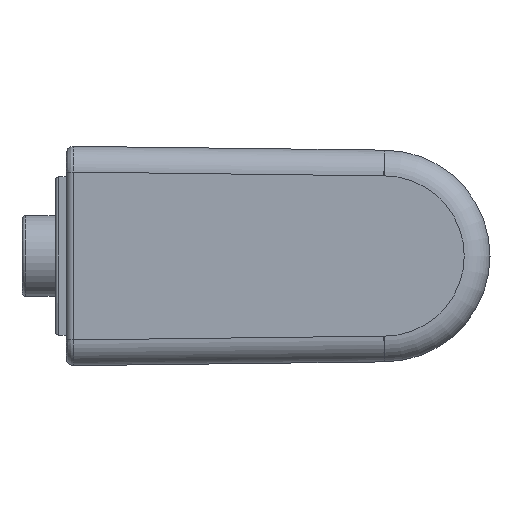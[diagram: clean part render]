
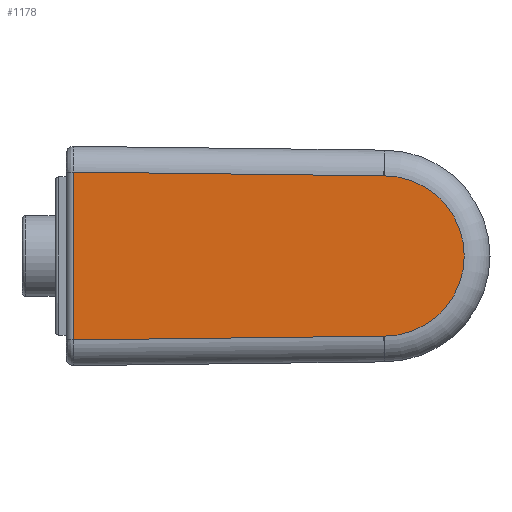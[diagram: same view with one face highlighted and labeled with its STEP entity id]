
A CAD part, left-side view. The second image highlights one B-rep face of the part: STEP entity #1178.
In plain terms, the highlighted planar face has unit normal (-1, 0, 0).
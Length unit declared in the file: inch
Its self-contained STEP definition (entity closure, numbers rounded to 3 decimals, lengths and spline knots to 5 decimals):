
#82 = ORIENTED_EDGE ( 'NONE', *, *, #93, .T. ) ;
#93 = EDGE_CURVE ( 'NONE', #394, #2567, #2109, .T. ) ;
#177 = EDGE_CURVE ( 'NONE', #1237, #2096, #2290, .T. ) ;
#301 = CARTESIAN_POINT ( 'NONE',  ( -9.35, 0., 0. ) ) ;
#338 = DIRECTION ( 'NONE',  ( 0., -1., 0.012 ) ) ;
#391 = CARTESIAN_POINT ( 'NONE',  ( -9.35, -0.02646, -2.17963 ) ) ;
#394 = VERTEX_POINT ( 'NONE', #2367 ) ;
#497 = PLANE ( 'NONE',  #523 ) ;
#521 = CARTESIAN_POINT ( 'NONE',  ( -9.35, -0.02646, 2.17963 ) ) ;
#523 = AXIS2_PLACEMENT_3D ( 'NONE', #2022, #2000, #2430 ) ;
#545 = ORIENTED_EDGE ( 'NONE', *, *, #1385, .T. ) ;
#581 = VERTEX_POINT ( 'NONE', #2071 ) ;
#717 = LINE ( 'NONE', #521, #2708 ) ;
#722 = EDGE_LOOP ( 'NONE', ( #1067, #1411, #984, #545, #1349, #82 ) ) ;
#735 = VECTOR ( 'NONE', #338, 39.37008 ) ;
#756 = VERTEX_POINT ( 'NONE', #1978 ) ;
#837 = DIRECTION ( 'NONE',  ( -1., 0., 0. ) ) ;
#890 = AXIS2_PLACEMENT_3D ( 'NONE', #2452, #2725, #1841 ) ;
#984 = ORIENTED_EDGE ( 'NONE', *, *, #2541, .T. ) ;
#1067 = ORIENTED_EDGE ( 'NONE', *, *, #2399, .T. ) ;
#1105 = CIRCLE ( 'NONE', #2674, 2.18 ) ;
#1151 = DIRECTION ( 'NONE',  ( -1., 0., 0. ) ) ;
#1178 = ADVANCED_FACE ( 'NONE', ( #1800 ), #497, .F. ) ;
#1182 = CARTESIAN_POINT ( 'NONE',  ( -9.35, 8.45, -2.28252 ) ) ;
#1234 = AXIS2_PLACEMENT_3D ( 'NONE', #301, #1151, #2453 ) ;
#1237 = VERTEX_POINT ( 'NONE', #2227 ) ;
#1243 = EDGE_CURVE ( 'NONE', #581, #394, #1421, .T. ) ;
#1252 = VECTOR ( 'NONE', #1615, 39.37008 ) ;
#1349 = ORIENTED_EDGE ( 'NONE', *, *, #1243, .T. ) ;
#1377 = DIRECTION ( 'NONE',  ( 0., 1., 0.012 ) ) ;
#1385 = EDGE_CURVE ( 'NONE', #756, #581, #1105, .T. ) ;
#1411 = ORIENTED_EDGE ( 'NONE', *, *, #177, .T. ) ;
#1421 = CIRCLE ( 'NONE', #1234, 2.18 ) ;
#1460 = LINE ( 'NONE', #391, #735 ) ;
#1527 = CARTESIAN_POINT ( 'NONE',  ( -9.35, 0., 0. ) ) ;
#1615 = DIRECTION ( 'NONE',  ( 0., 0., -1. ) ) ;
#1800 = FACE_OUTER_BOUND ( 'NONE', #722, .T. ) ;
#1841 = DIRECTION ( 'NONE',  ( 0., 0., -1. ) ) ;
#1978 = CARTESIAN_POINT ( 'NONE',  ( -9.35, 0.00395, -2.18 ) ) ;
#2000 = DIRECTION ( 'NONE',  ( 1., 0., 0. ) ) ;
#2022 = CARTESIAN_POINT ( 'NONE',  ( -9.35, 0., 0. ) ) ;
#2033 = CARTESIAN_POINT ( 'NONE',  ( -9.35, 8.45, 0. ) ) ;
#2071 = CARTESIAN_POINT ( 'NONE',  ( -9.35, 0., -2.18 ) ) ;
#2096 = VERTEX_POINT ( 'NONE', #1182 ) ;
#2106 = CARTESIAN_POINT ( 'NONE',  ( -9.35, 0.00395, 2.18 ) ) ;
#2109 = CIRCLE ( 'NONE', #890, 2.18 ) ;
#2151 = DIRECTION ( 'NONE',  ( 0., 0., -1. ) ) ;
#2227 = CARTESIAN_POINT ( 'NONE',  ( -9.35, 8.45, 2.28252 ) ) ;
#2290 = LINE ( 'NONE', #2033, #1252 ) ;
#2367 = CARTESIAN_POINT ( 'NONE',  ( -9.35, 0., 2.18 ) ) ;
#2399 = EDGE_CURVE ( 'NONE', #2567, #1237, #717, .T. ) ;
#2430 = DIRECTION ( 'NONE',  ( 0., 0., -1. ) ) ;
#2452 = CARTESIAN_POINT ( 'NONE',  ( -9.35, 0., 0. ) ) ;
#2453 = DIRECTION ( 'NONE',  ( 0., 0., -1. ) ) ;
#2541 = EDGE_CURVE ( 'NONE', #2096, #756, #1460, .T. ) ;
#2567 = VERTEX_POINT ( 'NONE', #2106 ) ;
#2674 = AXIS2_PLACEMENT_3D ( 'NONE', #1527, #837, #2151 ) ;
#2708 = VECTOR ( 'NONE', #1377, 39.37008 ) ;
#2725 = DIRECTION ( 'NONE',  ( -1., 0., 0. ) ) ;
